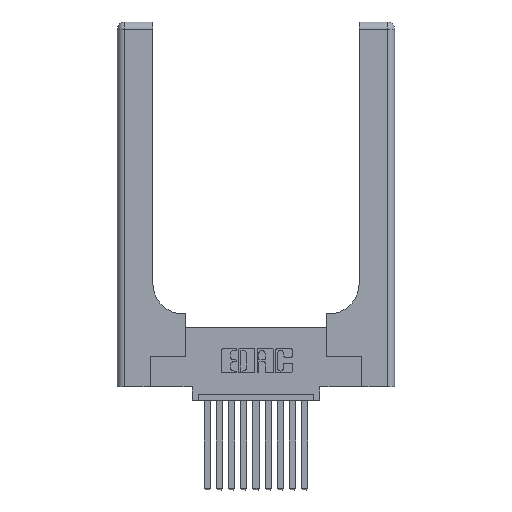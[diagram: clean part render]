
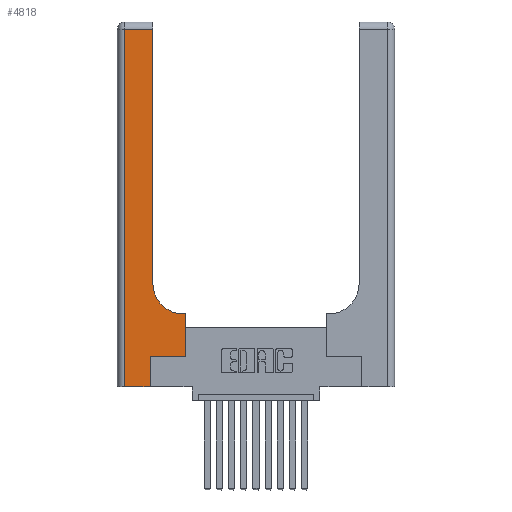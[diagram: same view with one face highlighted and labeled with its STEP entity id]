
A CAD part, top view. The second image highlights one B-rep face of the part: STEP entity #4818.
In plain terms, the highlighted planar face has unit normal (0, 0, 1).
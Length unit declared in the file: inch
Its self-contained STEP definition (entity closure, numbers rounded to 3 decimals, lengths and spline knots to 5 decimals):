
#16 = CARTESIAN_POINT ( 'NONE',  ( 0., 0., 0.37 ) ) ;
#97 = LINE ( 'NONE', #16, #9962 ) ;
#108 = VERTEX_POINT ( 'NONE', #10012 ) ;
#200 = ORIENTED_EDGE ( 'NONE', *, *, #7530, .T. ) ;
#269 = FACE_OUTER_BOUND ( 'NONE', #10418, .T. ) ;
#836 = CARTESIAN_POINT ( 'NONE',  ( 0., 3., 0.37 ) ) ;
#842 = DIRECTION ( 'NONE',  ( 0., 1., 0. ) ) ;
#857 = LINE ( 'NONE', #8890, #7969 ) ;
#1408 = VECTOR ( 'NONE', #13659, 39.37008 ) ;
#1958 = CARTESIAN_POINT ( 'NONE',  ( 0.5585, 0.25, 0.37 ) ) ;
#2084 = ORIENTED_EDGE ( 'NONE', *, *, #9629, .T. ) ;
#2373 = ORIENTED_EDGE ( 'NONE', *, *, #11799, .T. ) ;
#2548 = ORIENTED_EDGE ( 'NONE', *, *, #14031, .T. ) ;
#2561 = DIRECTION ( 'NONE',  ( 0., 1., 0. ) ) ;
#2670 = DIRECTION ( 'NONE',  ( 0., 0., -1. ) ) ;
#2959 = VERTEX_POINT ( 'NONE', #10016 ) ;
#3120 = DIRECTION ( 'NONE',  ( 0., 0., -1. ) ) ;
#3242 = VECTOR ( 'NONE', #2561, 39.37008 ) ;
#3348 = VERTEX_POINT ( 'NONE', #10448 ) ;
#3638 = DIRECTION ( 'NONE',  ( 1., 0., 0. ) ) ;
#3844 = DIRECTION ( 'NONE',  ( -1., 0., 0. ) ) ;
#3937 = ORIENTED_EDGE ( 'NONE', *, *, #15096, .T. ) ;
#3967 = VERTEX_POINT ( 'NONE', #11014 ) ;
#4140 = VECTOR ( 'NONE', #11663, 39.37008 ) ;
#4200 = CARTESIAN_POINT ( 'NONE',  ( 0.2915, 2.94, 0.37 ) ) ;
#4327 = LINE ( 'NONE', #8038, #12163 ) ;
#4419 = LINE ( 'NONE', #13413, #5395 ) ;
#4790 = ORIENTED_EDGE ( 'NONE', *, *, #10356, .T. ) ;
#4792 = LINE ( 'NONE', #15143, #11837 ) ;
#4818 = ADVANCED_FACE ( 'NONE', ( #269 ), #8346, .F. ) ;
#5395 = VECTOR ( 'NONE', #842, 39.37008 ) ;
#6317 = ORIENTED_EDGE ( 'NONE', *, *, #15051, .T. ) ;
#6330 = CARTESIAN_POINT ( 'NONE',  ( 0.269, 0., 0.37 ) ) ;
#6691 = LINE ( 'NONE', #10369, #4140 ) ;
#7102 = VERTEX_POINT ( 'NONE', #1958 ) ;
#7213 = CIRCLE ( 'NONE', #15111, 0.25 ) ;
#7530 = EDGE_CURVE ( 'NONE', #13211, #11433, #857, .T. ) ;
#7643 = DIRECTION ( 'NONE',  ( 1., 0., 0. ) ) ;
#7737 = DIRECTION ( 'NONE',  ( 1., 0., 0. ) ) ;
#7969 = VECTOR ( 'NONE', #3844, 39.37008 ) ;
#7988 = ORIENTED_EDGE ( 'NONE', *, *, #14351, .T. ) ;
#8038 = CARTESIAN_POINT ( 'NONE',  ( 0.2915, 0.6, 0.37 ) ) ;
#8346 = PLANE ( 'NONE',  #10924 ) ;
#8890 = CARTESIAN_POINT ( 'NONE',  ( 0., 2.94, 0.37 ) ) ;
#9231 = ORIENTED_EDGE ( 'NONE', *, *, #15849, .T. ) ;
#9629 = EDGE_CURVE ( 'NONE', #3967, #3348, #7213, .T. ) ;
#9962 = VECTOR ( 'NONE', #7643, 39.37008 ) ;
#10012 = CARTESIAN_POINT ( 'NONE',  ( 0.5585, 0.6, 0.37 ) ) ;
#10016 = CARTESIAN_POINT ( 'NONE',  ( 0.269, 0.25, 0.37 ) ) ;
#10167 = VERTEX_POINT ( 'NONE', #12525 ) ;
#10200 = CARTESIAN_POINT ( 'NONE',  ( 0.5415, 0.85, 0.37 ) ) ;
#10356 = EDGE_CURVE ( 'NONE', #108, #3967, #4327, .T. ) ;
#10369 = CARTESIAN_POINT ( 'NONE',  ( 0.06, 3., 0.37 ) ) ;
#10418 = EDGE_LOOP ( 'NONE', ( #2548, #200, #9231, #2373, #7988, #6317, #3937, #4790, #2084 ) ) ;
#10448 = CARTESIAN_POINT ( 'NONE',  ( 0.2915, 0.85, 0.37 ) ) ;
#10924 = AXIS2_PLACEMENT_3D ( 'NONE', #836, #3120, #11894 ) ;
#11014 = CARTESIAN_POINT ( 'NONE',  ( 0.5415, 0.6, 0.37 ) ) ;
#11433 = VERTEX_POINT ( 'NONE', #14098 ) ;
#11663 = DIRECTION ( 'NONE',  ( 0., -1., 0. ) ) ;
#11799 = EDGE_CURVE ( 'NONE', #10167, #16269, #97, .T. ) ;
#11837 = VECTOR ( 'NONE', #3638, 39.37008 ) ;
#11854 = LINE ( 'NONE', #15129, #3242 ) ;
#11894 = DIRECTION ( 'NONE',  ( -1., 0., 0. ) ) ;
#12163 = VECTOR ( 'NONE', #14249, 39.37008 ) ;
#12233 = LINE ( 'NONE', #12366, #1408 ) ;
#12366 = CARTESIAN_POINT ( 'NONE',  ( 0.5585, 0.25, 0.37 ) ) ;
#12525 = CARTESIAN_POINT ( 'NONE',  ( 0.06, 0., 0.37 ) ) ;
#13211 = VERTEX_POINT ( 'NONE', #4200 ) ;
#13413 = CARTESIAN_POINT ( 'NONE',  ( 0.269, 0., 0.37 ) ) ;
#13659 = DIRECTION ( 'NONE',  ( 0., 1., 0. ) ) ;
#14031 = EDGE_CURVE ( 'NONE', #3348, #13211, #11854, .T. ) ;
#14098 = CARTESIAN_POINT ( 'NONE',  ( 0.06, 2.94, 0.37 ) ) ;
#14249 = DIRECTION ( 'NONE',  ( -1., 0., 0. ) ) ;
#14351 = EDGE_CURVE ( 'NONE', #16269, #2959, #4419, .T. ) ;
#15051 = EDGE_CURVE ( 'NONE', #2959, #7102, #4792, .T. ) ;
#15096 = EDGE_CURVE ( 'NONE', #7102, #108, #12233, .T. ) ;
#15111 = AXIS2_PLACEMENT_3D ( 'NONE', #10200, #2670, #7737 ) ;
#15129 = CARTESIAN_POINT ( 'NONE',  ( 0.2915, 3., 0.37 ) ) ;
#15143 = CARTESIAN_POINT ( 'NONE',  ( 0.269, 0.25, 0.37 ) ) ;
#15849 = EDGE_CURVE ( 'NONE', #11433, #10167, #6691, .T. ) ;
#16269 = VERTEX_POINT ( 'NONE', #6330 ) ;
